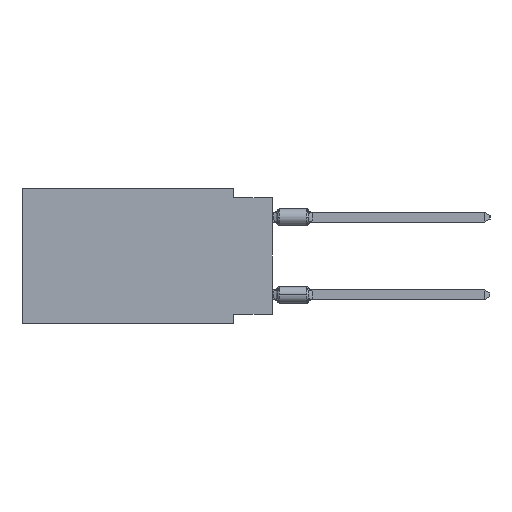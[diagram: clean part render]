
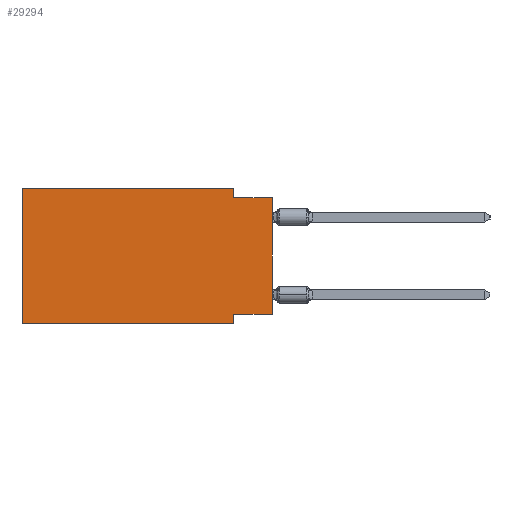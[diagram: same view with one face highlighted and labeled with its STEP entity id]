
A CAD part, left-side view. The second image highlights one B-rep face of the part: STEP entity #29294.
In plain terms, the highlighted planar face has unit normal (-1, 0, 0).
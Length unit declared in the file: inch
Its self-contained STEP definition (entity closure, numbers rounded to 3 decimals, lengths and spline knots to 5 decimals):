
#1420 = DIRECTION ( 'NONE',  ( 0., 1., 0. ) ) ;
#1831 = ORIENTED_EDGE ( 'NONE', *, *, #20530, .F. ) ;
#1886 = FACE_OUTER_BOUND ( 'NONE', #33127, .T. ) ;
#2612 = ORIENTED_EDGE ( 'NONE', *, *, #36871, .F. ) ;
#5490 = ORIENTED_EDGE ( 'NONE', *, *, #40482, .F. ) ;
#5904 = DIRECTION ( 'NONE',  ( 0., 0., 1. ) ) ;
#6246 = DIRECTION ( 'NONE',  ( 1., 0., 0. ) ) ;
#6545 = CARTESIAN_POINT ( 'NONE',  ( 0., 0.645, 0. ) ) ;
#6671 = CARTESIAN_POINT ( 'NONE',  ( 0., 0., 0. ) ) ;
#6894 = VECTOR ( 'NONE', #49599, 39.37008 ) ;
#7649 = DIRECTION ( 'NONE',  ( 0., -1., 0. ) ) ;
#8050 = VECTOR ( 'NONE', #18849, 39.37008 ) ;
#8080 = LINE ( 'NONE', #43129, #6894 ) ;
#9171 = ORIENTED_EDGE ( 'NONE', *, *, #25218, .T. ) ;
#10010 = CARTESIAN_POINT ( 'NONE',  ( 0., 0.1, -0.025 ) ) ;
#10524 = LINE ( 'NONE', #6671, #10767 ) ;
#10767 = VECTOR ( 'NONE', #5904, 39.37008 ) ;
#10803 = ORIENTED_EDGE ( 'NONE', *, *, #39237, .F. ) ;
#11279 = VERTEX_POINT ( 'NONE', #28516 ) ;
#14129 = CARTESIAN_POINT ( 'NONE',  ( 0., 0., -0.025 ) ) ;
#14286 = VERTEX_POINT ( 'NONE', #38856 ) ;
#15158 = EDGE_CURVE ( 'NONE', #47203, #11279, #8080, .T. ) ;
#15475 = VERTEX_POINT ( 'NONE', #10010 ) ;
#16378 = CARTESIAN_POINT ( 'NONE',  ( 0., 0.1, -0.325 ) ) ;
#17753 = PLANE ( 'NONE',  #36123 ) ;
#17783 = LINE ( 'NONE', #24752, #30730 ) ;
#18849 = DIRECTION ( 'NONE',  ( 0., 0., -1. ) ) ;
#20530 = EDGE_CURVE ( 'NONE', #15475, #43234, #48193, .T. ) ;
#22265 = VERTEX_POINT ( 'NONE', #26134 ) ;
#24752 = CARTESIAN_POINT ( 'NONE',  ( 0., 0., -0.325 ) ) ;
#25218 = EDGE_CURVE ( 'NONE', #40297, #43234, #10524, .T. ) ;
#25897 = ORIENTED_EDGE ( 'NONE', *, *, #15158, .F. ) ;
#26134 = CARTESIAN_POINT ( 'NONE',  ( 0., 0.1, 0. ) ) ;
#28040 = VERTEX_POINT ( 'NONE', #43130 ) ;
#28516 = CARTESIAN_POINT ( 'NONE',  ( 0., 0.1, -0.35 ) ) ;
#29294 = ADVANCED_FACE ( 'NONE', ( #1886 ), #17753, .F. ) ;
#29376 = VECTOR ( 'NONE', #48432, 39.37008 ) ;
#29841 = LINE ( 'NONE', #6545, #37350 ) ;
#30026 = ORIENTED_EDGE ( 'NONE', *, *, #45110, .F. ) ;
#30628 = CARTESIAN_POINT ( 'NONE',  ( 0., 0.645, 0. ) ) ;
#30730 = VECTOR ( 'NONE', #1420, 39.37008 ) ;
#30969 = CARTESIAN_POINT ( 'NONE',  ( 0., 0.645, -0.35 ) ) ;
#32882 = EDGE_CURVE ( 'NONE', #28040, #11279, #42712, .T. ) ;
#33127 = EDGE_LOOP ( 'NONE', ( #9171, #1831, #30026, #5490, #10803, #37744, #25897, #2612 ) ) ;
#34246 = LINE ( 'NONE', #30628, #48693 ) ;
#34505 = DIRECTION ( 'NONE',  ( 0., -1., 0. ) ) ;
#34609 = VECTOR ( 'NONE', #7649, 39.37008 ) ;
#35007 = LINE ( 'NONE', #38068, #8050 ) ;
#36123 = AXIS2_PLACEMENT_3D ( 'NONE', #41313, #6246, #44654 ) ;
#36871 = EDGE_CURVE ( 'NONE', #40297, #47203, #17783, .T. ) ;
#37350 = VECTOR ( 'NONE', #50293, 39.37008 ) ;
#37744 = ORIENTED_EDGE ( 'NONE', *, *, #32882, .T. ) ;
#38068 = CARTESIAN_POINT ( 'NONE',  ( 0., 0.1, 0. ) ) ;
#38856 = CARTESIAN_POINT ( 'NONE',  ( 0., 0.645, 0. ) ) ;
#39237 = EDGE_CURVE ( 'NONE', #28040, #14286, #29841, .T. ) ;
#39898 = CARTESIAN_POINT ( 'NONE',  ( 0., 0., -0.325 ) ) ;
#40297 = VERTEX_POINT ( 'NONE', #39898 ) ;
#40482 = EDGE_CURVE ( 'NONE', #14286, #22265, #34246, .T. ) ;
#41313 = CARTESIAN_POINT ( 'NONE',  ( 0., 0.645, 0. ) ) ;
#42712 = LINE ( 'NONE', #30969, #34609 ) ;
#43129 = CARTESIAN_POINT ( 'NONE',  ( 0., 0.1, -0.35 ) ) ;
#43130 = CARTESIAN_POINT ( 'NONE',  ( 0., 0.645, -0.35 ) ) ;
#43234 = VERTEX_POINT ( 'NONE', #47363 ) ;
#44654 = DIRECTION ( 'NONE',  ( 0., 0., -1. ) ) ;
#45110 = EDGE_CURVE ( 'NONE', #22265, #15475, #35007, .T. ) ;
#47203 = VERTEX_POINT ( 'NONE', #16378 ) ;
#47363 = CARTESIAN_POINT ( 'NONE',  ( 0., 0., -0.025 ) ) ;
#48193 = LINE ( 'NONE', #14129, #29376 ) ;
#48432 = DIRECTION ( 'NONE',  ( 0., -1., 0. ) ) ;
#48693 = VECTOR ( 'NONE', #34505, 39.37008 ) ;
#49599 = DIRECTION ( 'NONE',  ( 0., 0., -1. ) ) ;
#50293 = DIRECTION ( 'NONE',  ( 0., 0., 1. ) ) ;
